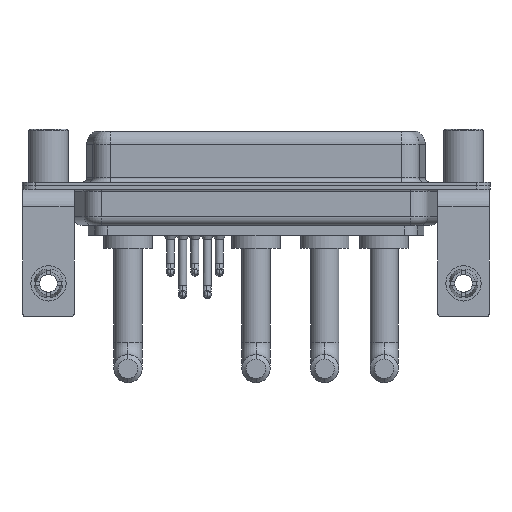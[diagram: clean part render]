
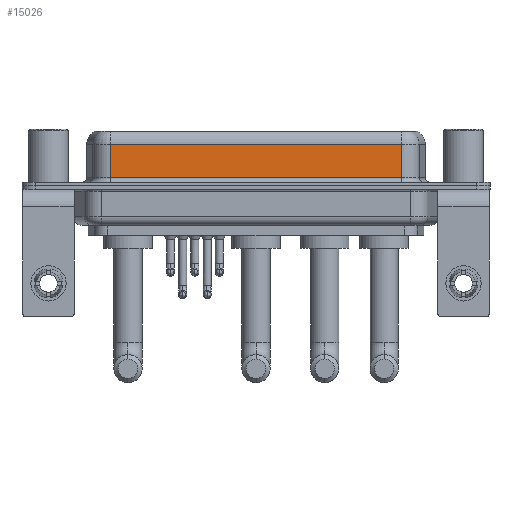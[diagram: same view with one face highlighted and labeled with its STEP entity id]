
A CAD part, front view. The second image highlights one B-rep face of the part: STEP entity #15026.
In plain terms, the highlighted planar face has unit normal (0, -1, 0).
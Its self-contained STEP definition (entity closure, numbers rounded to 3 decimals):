
#512 = EDGE_CURVE ( 'NONE', #17127, #5542, #7228, .T. ) ;
#593 = EDGE_CURVE ( 'NONE', #4952, #15339, #13951, .T. ) ;
#636 = DIRECTION ( 'NONE',  ( 0., 0., -1. ) ) ;
#946 = CARTESIAN_POINT ( 'NONE',  ( 7.013, -3.95, 4.65 ) ) ;
#1523 = CARTESIAN_POINT ( 'NONE',  ( 40.037, -3.95, 6.4 ) ) ;
#1744 = EDGE_CURVE ( 'NONE', #4952, #5542, #17941, .T. ) ;
#4952 = VERTEX_POINT ( 'NONE', #7525 ) ;
#5501 = ORIENTED_EDGE ( 'NONE', *, *, #13898, .T. ) ;
#5527 = LINE ( 'NONE', #14171, #16547 ) ;
#5542 = VERTEX_POINT ( 'NONE', #12297 ) ;
#6380 = CARTESIAN_POINT ( 'NONE',  ( 40.037, -3.95, 6.4 ) ) ;
#7228 = LINE ( 'NONE', #12319, #7353 ) ;
#7353 = VECTOR ( 'NONE', #15258, 1000. ) ;
#7525 = CARTESIAN_POINT ( 'NONE',  ( 40.037, -3.95, 4.65 ) ) ;
#7905 = PLANE ( 'NONE',  #11773 ) ;
#8220 = FACE_OUTER_BOUND ( 'NONE', #15025, .T. ) ;
#11042 = ORIENTED_EDGE ( 'NONE', *, *, #1744, .F. ) ;
#11773 = AXIS2_PLACEMENT_3D ( 'NONE', #1523, #14823, #16135 ) ;
#12009 = CARTESIAN_POINT ( 'NONE',  ( 40.037, -3.95, 4.65 ) ) ;
#12297 = CARTESIAN_POINT ( 'NONE',  ( 40.037, -3.95, 0.9 ) ) ;
#12319 = CARTESIAN_POINT ( 'NONE',  ( 40.037, -3.95, 0.9 ) ) ;
#13898 = EDGE_CURVE ( 'NONE', #15339, #17127, #5527, .T. ) ;
#13951 = LINE ( 'NONE', #12009, #21178 ) ;
#14171 = CARTESIAN_POINT ( 'NONE',  ( 7.013, -3.95, 6.4 ) ) ;
#14527 = ORIENTED_EDGE ( 'NONE', *, *, #593, .T. ) ;
#14823 = DIRECTION ( 'NONE',  ( 0., 1., 0. ) ) ;
#15025 = EDGE_LOOP ( 'NONE', ( #11042, #14527, #5501, #17848 ) ) ;
#15026 = ADVANCED_FACE ( 'NONE', ( #8220 ), #7905, .F. ) ;
#15258 = DIRECTION ( 'NONE',  ( 1., 0., 0. ) ) ;
#15339 = VERTEX_POINT ( 'NONE', #946 ) ;
#16135 = DIRECTION ( 'NONE',  ( 0., 0., 1. ) ) ;
#16547 = VECTOR ( 'NONE', #636, 1000. ) ;
#17127 = VERTEX_POINT ( 'NONE', #18160 ) ;
#17848 = ORIENTED_EDGE ( 'NONE', *, *, #512, .T. ) ;
#17941 = LINE ( 'NONE', #6380, #20288 ) ;
#18160 = CARTESIAN_POINT ( 'NONE',  ( 7.013, -3.95, 0.9 ) ) ;
#18693 = DIRECTION ( 'NONE',  ( -1., 0., 0. ) ) ;
#19235 = DIRECTION ( 'NONE',  ( 0., 0., -1. ) ) ;
#20288 = VECTOR ( 'NONE', #19235, 1000. ) ;
#21178 = VECTOR ( 'NONE', #18693, 1000. ) ;
